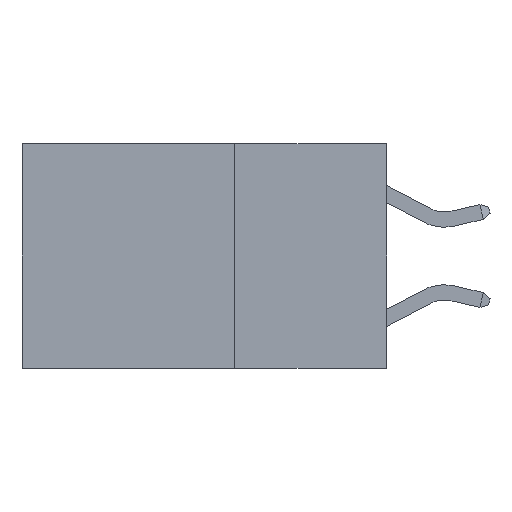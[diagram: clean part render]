
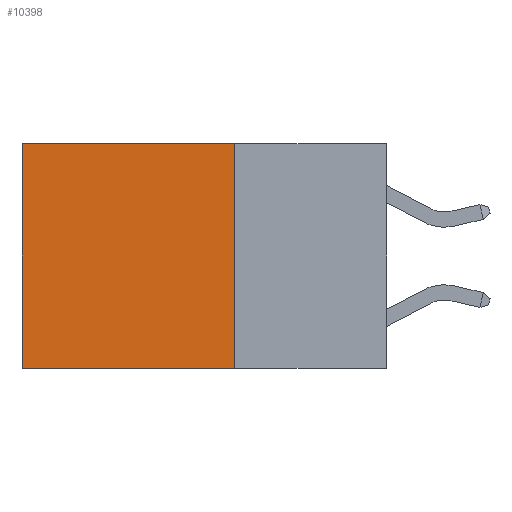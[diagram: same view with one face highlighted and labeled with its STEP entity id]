
A CAD part, left-side view. The second image highlights one B-rep face of the part: STEP entity #10398.
In plain terms, the highlighted planar face has unit normal (-1, 0, 0).
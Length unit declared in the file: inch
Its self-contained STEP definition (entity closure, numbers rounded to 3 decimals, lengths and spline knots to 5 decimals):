
#1196 = CARTESIAN_POINT ( 'NONE',  ( 0.2625, 0.25, 0. ) ) ;
#1253 = DIRECTION ( 'NONE',  ( 0., 0., -1. ) ) ;
#1936 = PLANE ( 'NONE',  #3555 ) ;
#2250 = DIRECTION ( 'NONE',  ( 0., 0., -1. ) ) ;
#2566 = VECTOR ( 'NONE', #2756, 39.37008 ) ;
#2756 = DIRECTION ( 'NONE',  ( 0., 1., 0. ) ) ;
#3555 = AXIS2_PLACEMENT_3D ( 'NONE', #13907, #6675, #13680 ) ;
#3619 = EDGE_CURVE ( 'NONE', #12570, #13992, #4551, .T. ) ;
#3633 = VECTOR ( 'NONE', #7003, 39.37008 ) ;
#4035 = EDGE_CURVE ( 'NONE', #4332, #8214, #11578, .T. ) ;
#4332 = VERTEX_POINT ( 'NONE', #13188 ) ;
#4551 = LINE ( 'NONE', #4761, #6714 ) ;
#4761 = CARTESIAN_POINT ( 'NONE',  ( 0.2625, 0.6, 0. ) ) ;
#5594 = LINE ( 'NONE', #12637, #3633 ) ;
#5757 = CARTESIAN_POINT ( 'NONE',  ( 0.2625, 0.6, 0. ) ) ;
#6568 = CARTESIAN_POINT ( 'NONE',  ( 0.2625, 0.6, -0.37 ) ) ;
#6675 = DIRECTION ( 'NONE',  ( 1., 0., 0. ) ) ;
#6714 = VECTOR ( 'NONE', #1253, 39.37008 ) ;
#6905 = EDGE_LOOP ( 'NONE', ( #8717, #11373, #11530, #12561 ) ) ;
#6973 = FACE_OUTER_BOUND ( 'NONE', #6905, .T. ) ;
#7003 = DIRECTION ( 'NONE',  ( 0., 1., 0. ) ) ;
#7450 = VECTOR ( 'NONE', #2250, 39.37008 ) ;
#8214 = VERTEX_POINT ( 'NONE', #10078 ) ;
#8717 = ORIENTED_EDGE ( 'NONE', *, *, #3619, .T. ) ;
#9939 = EDGE_CURVE ( 'NONE', #8214, #13992, #13350, .T. ) ;
#10078 = CARTESIAN_POINT ( 'NONE',  ( 0.2625, 0.25, -0.37 ) ) ;
#10398 = ADVANCED_FACE ( 'NONE', ( #6973 ), #1936, .F. ) ;
#11373 = ORIENTED_EDGE ( 'NONE', *, *, #9939, .F. ) ;
#11530 = ORIENTED_EDGE ( 'NONE', *, *, #4035, .F. ) ;
#11578 = LINE ( 'NONE', #1196, #7450 ) ;
#12069 = CARTESIAN_POINT ( 'NONE',  ( 0.2625, 0.25, -0.37 ) ) ;
#12561 = ORIENTED_EDGE ( 'NONE', *, *, #14726, .T. ) ;
#12570 = VERTEX_POINT ( 'NONE', #5757 ) ;
#12637 = CARTESIAN_POINT ( 'NONE',  ( 0.2625, 0.25, 0. ) ) ;
#13188 = CARTESIAN_POINT ( 'NONE',  ( 0.2625, 0.25, 0. ) ) ;
#13350 = LINE ( 'NONE', #12069, #2566 ) ;
#13680 = DIRECTION ( 'NONE',  ( 0., 0., -1. ) ) ;
#13907 = CARTESIAN_POINT ( 'NONE',  ( 0.2625, 0.25, 0. ) ) ;
#13992 = VERTEX_POINT ( 'NONE', #6568 ) ;
#14726 = EDGE_CURVE ( 'NONE', #4332, #12570, #5594, .T. ) ;
